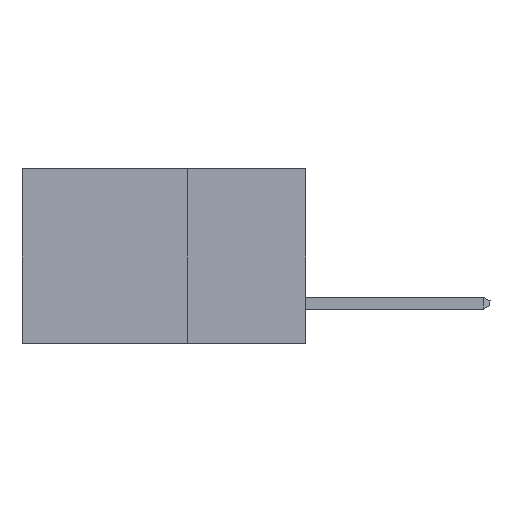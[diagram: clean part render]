
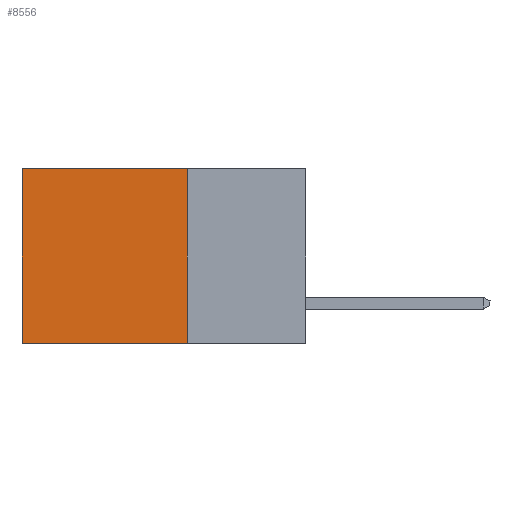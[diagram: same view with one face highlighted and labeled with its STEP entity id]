
A CAD part, left-side view. The second image highlights one B-rep face of the part: STEP entity #8556.
In plain terms, the highlighted planar face has unit normal (-1, 0, 0).
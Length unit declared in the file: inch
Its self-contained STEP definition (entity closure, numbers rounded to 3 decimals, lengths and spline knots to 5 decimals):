
#491 = CARTESIAN_POINT ( 'NONE',  ( 0.2615, 0.6, -0.37 ) ) ;
#803 = LINE ( 'NONE', #15968, #1603 ) ;
#1174 = EDGE_LOOP ( 'NONE', ( #22507, #10027, #17180, #14506 ) ) ;
#1603 = VECTOR ( 'NONE', #14047, 39.37008 ) ;
#1750 = LINE ( 'NONE', #9040, #4665 ) ;
#2088 = CARTESIAN_POINT ( 'NONE',  ( 0.2615, 0.6, 0. ) ) ;
#2312 = CARTESIAN_POINT ( 'NONE',  ( 0.2615, 0.6, -0.37 ) ) ;
#4665 = VECTOR ( 'NONE', #22343, 39.37008 ) ;
#7434 = EDGE_CURVE ( 'NONE', #17088, #14115, #7753, .T. ) ;
#7753 = LINE ( 'NONE', #491, #24176 ) ;
#7813 = CARTESIAN_POINT ( 'NONE',  ( 0.2615, 0.25, -0.37 ) ) ;
#7830 = VERTEX_POINT ( 'NONE', #21106 ) ;
#8556 = ADVANCED_FACE ( 'NONE', ( #11844 ), #15460, .F. ) ;
#9040 = CARTESIAN_POINT ( 'NONE',  ( 0.2615, 0.25, -0.37 ) ) ;
#9823 = DIRECTION ( 'NONE',  ( 1., 0., 0. ) ) ;
#10027 = ORIENTED_EDGE ( 'NONE', *, *, #20848, .F. ) ;
#11844 = FACE_OUTER_BOUND ( 'NONE', #1174, .T. ) ;
#14047 = DIRECTION ( 'NONE',  ( 0., 1., 0. ) ) ;
#14115 = VERTEX_POINT ( 'NONE', #2312 ) ;
#14506 = ORIENTED_EDGE ( 'NONE', *, *, #23924, .T. ) ;
#15460 = PLANE ( 'NONE',  #23058 ) ;
#15968 = CARTESIAN_POINT ( 'NONE',  ( 0.2615, 0.25, -0.37 ) ) ;
#17088 = VERTEX_POINT ( 'NONE', #2088 ) ;
#17180 = ORIENTED_EDGE ( 'NONE', *, *, #18163, .F. ) ;
#17470 = DIRECTION ( 'NONE',  ( 0., 0., -1. ) ) ;
#17525 = DIRECTION ( 'NONE',  ( 0., 0., -1. ) ) ;
#18163 = EDGE_CURVE ( 'NONE', #7830, #20478, #1750, .T. ) ;
#20478 = VERTEX_POINT ( 'NONE', #7813 ) ;
#20848 = EDGE_CURVE ( 'NONE', #20478, #14115, #803, .T. ) ;
#21106 = CARTESIAN_POINT ( 'NONE',  ( 0.2615, 0.25, 0. ) ) ;
#21862 = LINE ( 'NONE', #24074, #23515 ) ;
#22230 = DIRECTION ( 'NONE',  ( 0., 1., 0. ) ) ;
#22343 = DIRECTION ( 'NONE',  ( 0., 0., -1. ) ) ;
#22507 = ORIENTED_EDGE ( 'NONE', *, *, #7434, .T. ) ;
#23013 = CARTESIAN_POINT ( 'NONE',  ( 0.2615, 0.25, -0.37 ) ) ;
#23058 = AXIS2_PLACEMENT_3D ( 'NONE', #23013, #9823, #17470 ) ;
#23515 = VECTOR ( 'NONE', #22230, 39.37008 ) ;
#23924 = EDGE_CURVE ( 'NONE', #7830, #17088, #21862, .T. ) ;
#24074 = CARTESIAN_POINT ( 'NONE',  ( 0.2615, 0.25, 0. ) ) ;
#24176 = VECTOR ( 'NONE', #17525, 39.37008 ) ;
